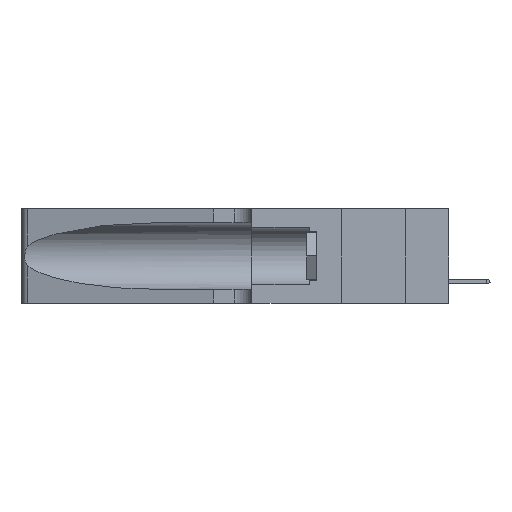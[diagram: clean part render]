
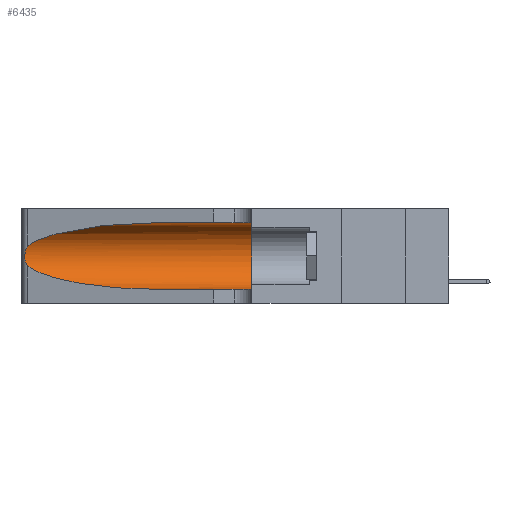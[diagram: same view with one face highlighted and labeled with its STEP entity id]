
A CAD part, left-side view. The second image highlights one B-rep face of the part: STEP entity #6435.
In plain terms, the highlighted cylindrical face has radius 3.308 mm (diameter 6.617 mm), a partial arc.
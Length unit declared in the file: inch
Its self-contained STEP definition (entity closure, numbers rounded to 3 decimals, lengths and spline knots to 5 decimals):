
#434 = CARTESIAN_POINT ( 'NONE',  ( 0.25487, 1.22718, 0.14631 ) ) ;
#647 = EDGE_CURVE ( 'NONE', #3260, #686, #17124, .T. ) ;
#686 = VERTEX_POINT ( 'NONE', #29619 ) ;
#1096 = CARTESIAN_POINT ( 'NONE',  ( 0.1305, 0.72297, 0.31525 ) ) ;
#2242 = VERTEX_POINT ( 'NONE', #11158 ) ;
#2631 = VERTEX_POINT ( 'NONE', #39377 ) ;
#3260 = VERTEX_POINT ( 'NONE', #26016 ) ;
#3481 = CARTESIAN_POINT ( 'NONE',  ( 0.25639, 1.23184, 0.21858 ) ) ;
#4154 = VERTEX_POINT ( 'NONE', #4530 ) ;
#4530 = CARTESIAN_POINT ( 'NONE',  ( 0.1305, 0.35, 0.05475 ) ) ;
#4679 = VERTEX_POINT ( 'NONE', #37756 ) ;
#6435 = ADVANCED_FACE ( 'NONE', ( #21154 ), #36555, .F. ) ;
#6652 = LINE ( 'NONE', #39507, #29172 ) ;
#6678 = CARTESIAN_POINT ( 'NONE',  ( 0.26017, 1.23833, 0.17102 ) ) ;
#7390 = CIRCLE ( 'NONE', #29503, 0.13025 ) ;
#7823 = DIRECTION ( 'NONE',  ( 0., -1., 0. ) ) ;
#8528 = CARTESIAN_POINT ( 'NONE',  ( 0.25487, 1.22718, 0.22369 ) ) ;
#8873 = CARTESIAN_POINT ( 'NONE',  ( 0.2373, 1.15595, 0.28018 ) ) ;
#9404 = CARTESIAN_POINT ( 'NONE',  ( 0.25787, 1.23484, 0.2124 ) ) ;
#9773 = ORIENTED_EDGE ( 'NONE', *, *, #14146, .F. ) ;
#9961 = ORIENTED_EDGE ( 'NONE', *, *, #10136, .T. ) ;
#10136 = EDGE_CURVE ( 'NONE', #4679, #4154, #6652, .T. ) ;
#10888 = LINE ( 'NONE', #14493, #40934 ) ;
#11158 = CARTESIAN_POINT ( 'NONE',  ( 0.1305, 0.72297, 0.31525 ) ) ;
#13586 = DIRECTION ( 'NONE',  ( 0., -1., 0. ) ) ;
#14146 = EDGE_CURVE ( 'NONE', #2242, #2631, #10888, .T. ) ;
#14493 = CARTESIAN_POINT ( 'NONE',  ( 0.1305, 1.61858, 0.31525 ) ) ;
#14688 = ORIENTED_EDGE ( 'NONE', *, *, #27024, .F. ) ;
#15733 = CARTESIAN_POINT ( 'NONE',  ( 0.25555, 1.22993, 0.14849 ) ) ;
#16770 = ORIENTED_EDGE ( 'NONE', *, *, #38920, .T. ) ;
#16786 = CARTESIAN_POINT ( 'NONE',  ( 0.25487, 1.22718, 0.14631 ) ) ;
#17124 = B_SPLINE_CURVE_WITH_KNOTS ( 'NONE', 3,
 ( #38590, #22657, #3481, #9404, #28816, #25856, #38192, #22403, #6678, #29068, #41298, #31629, #15733, #16786 ),
 .UNSPECIFIED., .F., .F.,
 ( 4, 2, 2, 2, 2, 2, 4 ),
 ( 0., 0.00027, 0.00053, 0.00107, 0.0016, 0.00187, 0.00214 ),
 .UNSPECIFIED. ) ;
#19321 = EDGE_LOOP ( 'NONE', ( #16770, #40804, #34000, #9961, #14688, #9773 ) ) ;
#19453 = CARTESIAN_POINT ( 'NONE',  ( 0.18966, 0.96281, 0.05475 ) ) ;
#21154 = FACE_OUTER_BOUND ( 'NONE', #19321, .T. ) ;
#22279 = CARTESIAN_POINT ( 'NONE',  ( 0.1305, 0.35, 0.185 ) ) ;
#22403 = CARTESIAN_POINT ( 'NONE',  ( 0.26075, 1.23896, 0.178 ) ) ;
#22657 = CARTESIAN_POINT ( 'NONE',  ( 0.25555, 1.22994, 0.2215 ) ) ;
#22846 = AXIS2_PLACEMENT_3D ( 'NONE', #32571, #13586, #29515 ) ;
#23681 = DIRECTION ( 'NONE',  ( 0., -1., 0. ) ) ;
#25856 = CARTESIAN_POINT ( 'NONE',  ( 0.26018, 1.23835, 0.19895 ) ) ;
#26016 = CARTESIAN_POINT ( 'NONE',  ( 0.25487, 1.22718, 0.22369 ) ) ;
#27024 = EDGE_CURVE ( 'NONE', #2631, #4154, #7390, .T. ) ;
#28678 = DIRECTION ( 'NONE',  ( 0., 1., 0. ) ) ;
#28816 = CARTESIAN_POINT ( 'NONE',  ( 0.25854, 1.2359, 0.20912 ) ) ;
#29068 = CARTESIAN_POINT ( 'NONE',  ( 0.25856, 1.23593, 0.16098 ) ) ;
#29172 = VECTOR ( 'NONE', #7823, 39.37008 ) ;
#29503 = AXIS2_PLACEMENT_3D ( 'NONE', #22279, #28678, #31875 ) ;
#29515 = DIRECTION ( 'NONE',  ( 0., 0., -1. ) ) ;
#29619 = CARTESIAN_POINT ( 'NONE',  ( 0.25487, 1.22718, 0.14631 ) ) ;
#29624 = CARTESIAN_POINT ( 'NONE',  ( 0.2373, 1.15595, 0.08982 ) ) ;
#29900 =( BOUNDED_CURVE ( )  B_SPLINE_CURVE ( 3, ( #434, #29624, #19453, #35333 ),
 .UNSPECIFIED., .F., .F. ) 
 B_SPLINE_CURVE_WITH_KNOTS ( ( 4, 4 ),
 ( 3.44316, 4.71239 ),
 .UNSPECIFIED. ) 
 CURVE ( )  GEOMETRIC_REPRESENTATION_ITEM ( )  RATIONAL_B_SPLINE_CURVE ( ( 1., 0.87, 0.87, 1. ) ) 
 REPRESENTATION_ITEM ( '' )  );
#31629 = CARTESIAN_POINT ( 'NONE',  ( 0.25639, 1.23186, 0.15144 ) ) ;
#31708 =( BOUNDED_CURVE ( )  B_SPLINE_CURVE ( 3, ( #1096, #33077, #8873, #8528 ),
 .UNSPECIFIED., .F., .T. ) 
 B_SPLINE_CURVE_WITH_KNOTS ( ( 4, 4 ),
 ( 1.5708, 2.84003 ),
 .UNSPECIFIED. ) 
 CURVE ( )  GEOMETRIC_REPRESENTATION_ITEM ( )  RATIONAL_B_SPLINE_CURVE ( ( 1., 0.87, 0.87, 1. ) ) 
 REPRESENTATION_ITEM ( '' )  );
#31875 = DIRECTION ( 'NONE',  ( 0., 0., 1. ) ) ;
#32571 = CARTESIAN_POINT ( 'NONE',  ( 0.1305, 1.61858, 0.185 ) ) ;
#33077 = CARTESIAN_POINT ( 'NONE',  ( 0.18966, 0.96281, 0.31525 ) ) ;
#34000 = ORIENTED_EDGE ( 'NONE', *, *, #37301, .T. ) ;
#35333 = CARTESIAN_POINT ( 'NONE',  ( 0.1305, 0.72297, 0.05475 ) ) ;
#36555 = CYLINDRICAL_SURFACE ( 'NONE', #22846, 0.13025 ) ;
#37301 = EDGE_CURVE ( 'NONE', #686, #4679, #29900, .T. ) ;
#37756 = CARTESIAN_POINT ( 'NONE',  ( 0.1305, 0.72297, 0.05475 ) ) ;
#38192 = CARTESIAN_POINT ( 'NONE',  ( 0.26075, 1.23896, 0.19203 ) ) ;
#38590 = CARTESIAN_POINT ( 'NONE',  ( 0.25487, 1.22718, 0.22369 ) ) ;
#38920 = EDGE_CURVE ( 'NONE', #2242, #3260, #31708, .T. ) ;
#39377 = CARTESIAN_POINT ( 'NONE',  ( 0.1305, 0.35, 0.31525 ) ) ;
#39507 = CARTESIAN_POINT ( 'NONE',  ( 0.1305, 1.61858, 0.05475 ) ) ;
#40804 = ORIENTED_EDGE ( 'NONE', *, *, #647, .T. ) ;
#40934 = VECTOR ( 'NONE', #23681, 39.37008 ) ;
#41298 = CARTESIAN_POINT ( 'NONE',  ( 0.25789, 1.23486, 0.15765 ) ) ;
